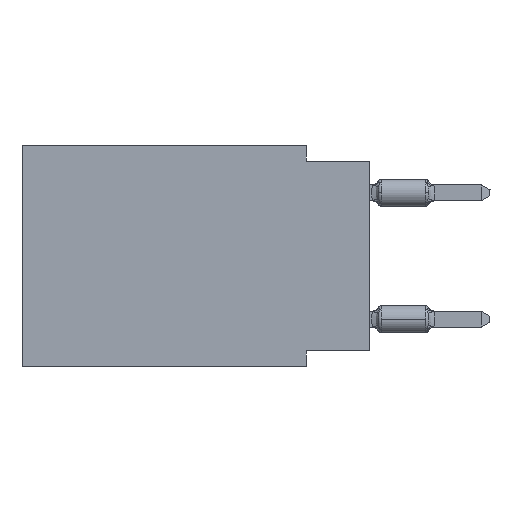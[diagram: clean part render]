
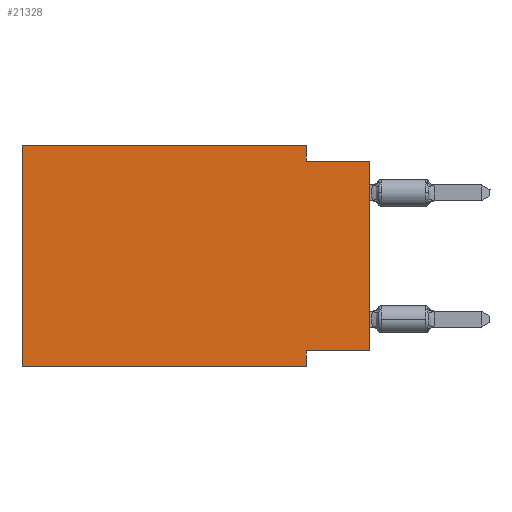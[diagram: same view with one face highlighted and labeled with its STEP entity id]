
A CAD part, left-side view. The second image highlights one B-rep face of the part: STEP entity #21328.
In plain terms, the highlighted planar face has unit normal (-1, 0, 0).
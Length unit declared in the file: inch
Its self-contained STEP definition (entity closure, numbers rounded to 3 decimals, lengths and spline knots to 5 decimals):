
#1753 = CARTESIAN_POINT ( 'NONE',  ( 0., 0.1, -0.35 ) ) ;
#5037 = EDGE_CURVE ( 'NONE', #53039, #33283, #16389, .T. ) ;
#5472 = LINE ( 'NONE', #17894, #55276 ) ;
#6443 = ORIENTED_EDGE ( 'NONE', *, *, #17415, .F. ) ;
#7882 = DIRECTION ( 'NONE',  ( 0., 1., 0. ) ) ;
#7967 = DIRECTION ( 'NONE',  ( 0., -1., 0. ) ) ;
#8637 = VERTEX_POINT ( 'NONE', #19538 ) ;
#10218 = VERTEX_POINT ( 'NONE', #46784 ) ;
#10953 = FACE_OUTER_BOUND ( 'NONE', #53940, .T. ) ;
#11032 = ORIENTED_EDGE ( 'NONE', *, *, #18413, .T. ) ;
#11216 = DIRECTION ( 'NONE',  ( 0., 0., 1. ) ) ;
#11503 = LINE ( 'NONE', #16361, #41112 ) ;
#12182 = EDGE_CURVE ( 'NONE', #10218, #57601, #31480, .T. ) ;
#12848 = VECTOR ( 'NONE', #11216, 39.37008 ) ;
#14280 = CARTESIAN_POINT ( 'NONE',  ( 0., 0.1, -0.35 ) ) ;
#14813 = ORIENTED_EDGE ( 'NONE', *, *, #49714, .F. ) ;
#15147 = EDGE_CURVE ( 'NONE', #22518, #40411, #11503, .T. ) ;
#15469 = CARTESIAN_POINT ( 'NONE',  ( 0., 0.55, 0. ) ) ;
#15525 = CARTESIAN_POINT ( 'NONE',  ( 0., 0., -0.025 ) ) ;
#16361 = CARTESIAN_POINT ( 'NONE',  ( 0., 0.55, 0. ) ) ;
#16389 = LINE ( 'NONE', #35739, #58074 ) ;
#17415 = EDGE_CURVE ( 'NONE', #33283, #32729, #48118, .T. ) ;
#17836 = DIRECTION ( 'NONE',  ( 0., 0., 1. ) ) ;
#17894 = CARTESIAN_POINT ( 'NONE',  ( 0., 0.1, 0. ) ) ;
#18413 = EDGE_CURVE ( 'NONE', #53039, #57601, #59032, .T. ) ;
#19538 = CARTESIAN_POINT ( 'NONE',  ( 0., 0.55, -0.35 ) ) ;
#21328 = ADVANCED_FACE ( 'NONE', ( #10953 ), #29422, .F. ) ;
#22387 = CARTESIAN_POINT ( 'NONE',  ( 0., 0., 0. ) ) ;
#22518 = VERTEX_POINT ( 'NONE', #42254 ) ;
#25094 = CARTESIAN_POINT ( 'NONE',  ( 0., 0.1, -0.325 ) ) ;
#27351 = CARTESIAN_POINT ( 'NONE',  ( 0., 0.55, -0.35 ) ) ;
#28218 = ORIENTED_EDGE ( 'NONE', *, *, #5037, .F. ) ;
#28251 = VECTOR ( 'NONE', #45438, 39.37008 ) ;
#29422 = PLANE ( 'NONE',  #44416 ) ;
#29607 = DIRECTION ( 'NONE',  ( 0., 0., -1. ) ) ;
#29685 = LINE ( 'NONE', #15469, #12848 ) ;
#31480 = LINE ( 'NONE', #49976, #28251 ) ;
#32729 = VERTEX_POINT ( 'NONE', #14280 ) ;
#33283 = VERTEX_POINT ( 'NONE', #25094 ) ;
#35739 = CARTESIAN_POINT ( 'NONE',  ( 0., 0., -0.325 ) ) ;
#35978 = VECTOR ( 'NONE', #7967, 39.37008 ) ;
#37856 = CARTESIAN_POINT ( 'NONE',  ( 0., 0., -0.325 ) ) ;
#39068 = DIRECTION ( 'NONE',  ( 0., -1., 0. ) ) ;
#40411 = VERTEX_POINT ( 'NONE', #49795 ) ;
#40681 = LINE ( 'NONE', #27351, #35978 ) ;
#41112 = VECTOR ( 'NONE', #39068, 39.37008 ) ;
#42254 = CARTESIAN_POINT ( 'NONE',  ( 0., 0.55, 0. ) ) ;
#43379 = DIRECTION ( 'NONE',  ( 0., 0., -1. ) ) ;
#43955 = CARTESIAN_POINT ( 'NONE',  ( 0., 0.55, 0. ) ) ;
#44416 = AXIS2_PLACEMENT_3D ( 'NONE', #43955, #48230, #43379 ) ;
#45438 = DIRECTION ( 'NONE',  ( 0., -1., 0. ) ) ;
#46154 = ORIENTED_EDGE ( 'NONE', *, *, #52360, .T. ) ;
#46784 = CARTESIAN_POINT ( 'NONE',  ( 0., 0.1, -0.025 ) ) ;
#46988 = VECTOR ( 'NONE', #29607, 39.37008 ) ;
#48118 = LINE ( 'NONE', #1753, #46988 ) ;
#48230 = DIRECTION ( 'NONE',  ( 1., 0., 0. ) ) ;
#49182 = ORIENTED_EDGE ( 'NONE', *, *, #15147, .F. ) ;
#49516 = ORIENTED_EDGE ( 'NONE', *, *, #12182, .F. ) ;
#49714 = EDGE_CURVE ( 'NONE', #40411, #10218, #5472, .T. ) ;
#49795 = CARTESIAN_POINT ( 'NONE',  ( 0., 0.1, 0. ) ) ;
#49976 = CARTESIAN_POINT ( 'NONE',  ( 0., 0., -0.025 ) ) ;
#51034 = EDGE_CURVE ( 'NONE', #8637, #22518, #29685, .T. ) ;
#51854 = VECTOR ( 'NONE', #17836, 39.37008 ) ;
#52360 = EDGE_CURVE ( 'NONE', #8637, #32729, #40681, .T. ) ;
#52478 = ORIENTED_EDGE ( 'NONE', *, *, #51034, .F. ) ;
#53039 = VERTEX_POINT ( 'NONE', #37856 ) ;
#53940 = EDGE_LOOP ( 'NONE', ( #11032, #49516, #14813, #49182, #52478, #46154, #6443, #28218 ) ) ;
#54866 = DIRECTION ( 'NONE',  ( 0., 0., -1. ) ) ;
#55276 = VECTOR ( 'NONE', #54866, 39.37008 ) ;
#57601 = VERTEX_POINT ( 'NONE', #15525 ) ;
#58074 = VECTOR ( 'NONE', #7882, 39.37008 ) ;
#59032 = LINE ( 'NONE', #22387, #51854 ) ;
